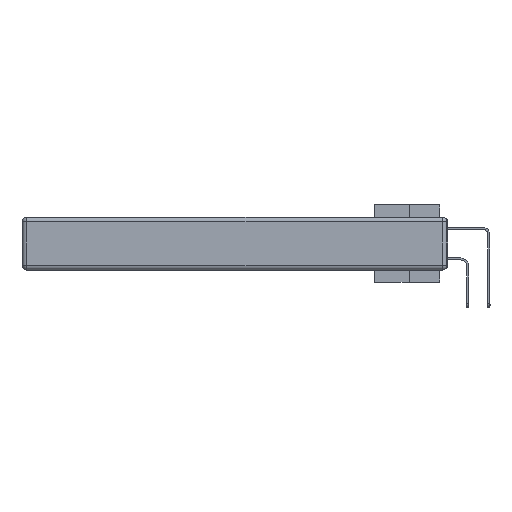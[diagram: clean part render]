
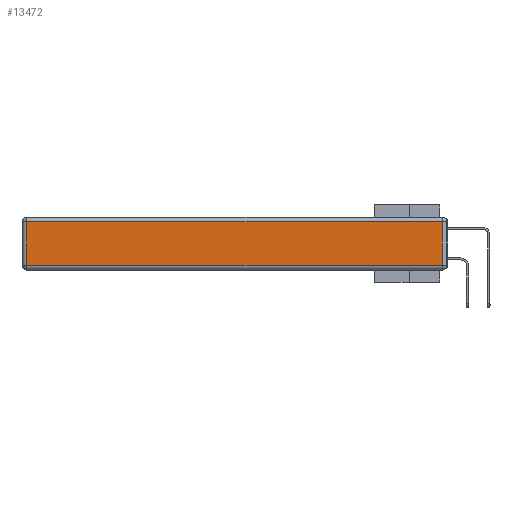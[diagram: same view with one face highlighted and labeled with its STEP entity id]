
A CAD part, left-side view. The second image highlights one B-rep face of the part: STEP entity #13472.
In plain terms, the highlighted planar face has unit normal (-1, 0, 0).
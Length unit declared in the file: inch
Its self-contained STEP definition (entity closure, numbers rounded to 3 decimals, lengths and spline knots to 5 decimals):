
#5062 = CARTESIAN_POINT ( 'NONE',  ( 0., 0.03, -0.03 ) ) ;
#5297 = VERTEX_POINT ( 'NONE', #6369 ) ;
#5728 = VECTOR ( 'NONE', #16842, 39.37008 ) ;
#6369 = CARTESIAN_POINT ( 'NONE',  ( 0., 2.72, -0.03 ) ) ;
#6812 = ORIENTED_EDGE ( 'NONE', *, *, #6858, .T. ) ;
#6858 = EDGE_CURVE ( 'NONE', #22562, #33467, #15178, .T. ) ;
#8797 = CARTESIAN_POINT ( 'NONE',  ( 0., 0.03, -0.313 ) ) ;
#9006 = CARTESIAN_POINT ( 'NONE',  ( 0., 2.72, -0.313 ) ) ;
#9286 = DIRECTION ( 'NONE',  ( 0., 0., 1. ) ) ;
#9369 = LINE ( 'NONE', #10118, #12260 ) ;
#10118 = CARTESIAN_POINT ( 'NONE',  ( 0., 2.75, -0.03 ) ) ;
#11141 = DIRECTION ( 'NONE',  ( 0., -1., 0. ) ) ;
#12050 = EDGE_CURVE ( 'NONE', #5297, #18671, #24955, .T. ) ;
#12260 = VECTOR ( 'NONE', #15365, 39.37008 ) ;
#13079 = VECTOR ( 'NONE', #11141, 39.37008 ) ;
#13472 = ADVANCED_FACE ( 'NONE', ( #33765 ), #22915, .T. ) ;
#14675 = EDGE_CURVE ( 'NONE', #33467, #5297, #9369, .T. ) ;
#14987 = CARTESIAN_POINT ( 'NONE',  ( 0., 0., -0.343 ) ) ;
#15068 = EDGE_CURVE ( 'NONE', #18671, #22562, #25214, .T. ) ;
#15178 = LINE ( 'NONE', #15343, #28569 ) ;
#15343 = CARTESIAN_POINT ( 'NONE',  ( 0., 0.03, -0.343 ) ) ;
#15365 = DIRECTION ( 'NONE',  ( 0., 1., 0. ) ) ;
#16842 = DIRECTION ( 'NONE',  ( 0., 0., -1. ) ) ;
#18671 = VERTEX_POINT ( 'NONE', #9006 ) ;
#19928 = DIRECTION ( 'NONE',  ( -1., 0., 0. ) ) ;
#22562 = VERTEX_POINT ( 'NONE', #8797 ) ;
#22915 = PLANE ( 'NONE',  #30349 ) ;
#23381 = ORIENTED_EDGE ( 'NONE', *, *, #14675, .T. ) ;
#23886 = ORIENTED_EDGE ( 'NONE', *, *, #15068, .T. ) ;
#24955 = LINE ( 'NONE', #27226, #5728 ) ;
#25214 = LINE ( 'NONE', #32473, #13079 ) ;
#26095 = ORIENTED_EDGE ( 'NONE', *, *, #12050, .T. ) ;
#27226 = CARTESIAN_POINT ( 'NONE',  ( 0., 2.72, -0.343 ) ) ;
#27284 = EDGE_LOOP ( 'NONE', ( #23886, #6812, #23381, #26095 ) ) ;
#28569 = VECTOR ( 'NONE', #28672, 39.37008 ) ;
#28672 = DIRECTION ( 'NONE',  ( 0., 0., 1. ) ) ;
#30349 = AXIS2_PLACEMENT_3D ( 'NONE', #14987, #19928, #9286 ) ;
#32473 = CARTESIAN_POINT ( 'NONE',  ( 0., 0., -0.313 ) ) ;
#33467 = VERTEX_POINT ( 'NONE', #5062 ) ;
#33765 = FACE_OUTER_BOUND ( 'NONE', #27284, .T. ) ;
